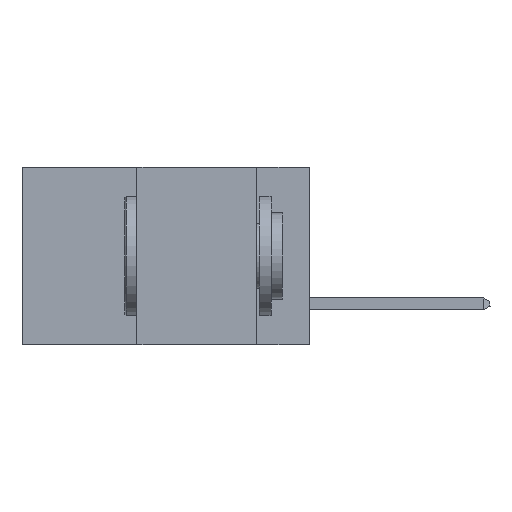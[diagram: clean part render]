
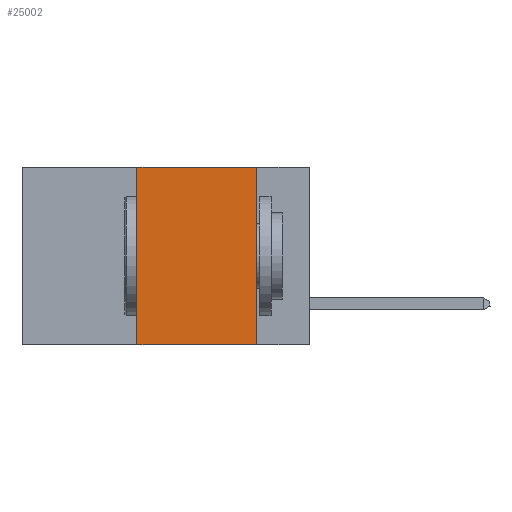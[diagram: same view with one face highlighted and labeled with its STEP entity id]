
A CAD part, left-side view. The second image highlights one B-rep face of the part: STEP entity #25002.
In plain terms, the highlighted planar face has unit normal (-1, 0, 0).
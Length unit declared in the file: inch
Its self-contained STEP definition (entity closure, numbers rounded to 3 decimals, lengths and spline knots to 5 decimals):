
#466 = CARTESIAN_POINT ( 'NONE',  ( 0., 0.6, 0. ) ) ;
#762 = VECTOR ( 'NONE', #21141, 39.37008 ) ;
#1636 = DIRECTION ( 'NONE',  ( 1., 0., 0. ) ) ;
#2012 = VERTEX_POINT ( 'NONE', #11096 ) ;
#3302 = ORIENTED_EDGE ( 'NONE', *, *, #7545, .F. ) ;
#3413 = ORIENTED_EDGE ( 'NONE', *, *, #18417, .F. ) ;
#3528 = VERTEX_POINT ( 'NONE', #21052 ) ;
#3825 = VERTEX_POINT ( 'NONE', #20026 ) ;
#4004 = CARTESIAN_POINT ( 'NONE',  ( 0., 0.6, -0.37 ) ) ;
#4723 = EDGE_LOOP ( 'NONE', ( #3302, #3413, #19471, #14823 ) ) ;
#5394 = LINE ( 'NONE', #10387, #23018 ) ;
#5799 = CARTESIAN_POINT ( 'NONE',  ( 0., 0.6, 0. ) ) ;
#7004 = VECTOR ( 'NONE', #17244, 39.37008 ) ;
#7545 = EDGE_CURVE ( 'NONE', #3528, #3825, #5394, .T. ) ;
#8318 = EDGE_CURVE ( 'NONE', #12825, #2012, #14344, .T. ) ;
#10387 = CARTESIAN_POINT ( 'NONE',  ( 0., 0.11, 0. ) ) ;
#10686 = CARTESIAN_POINT ( 'NONE',  ( 0., 0.36, 0. ) ) ;
#11096 = CARTESIAN_POINT ( 'NONE',  ( 0., 0.36, 0. ) ) ;
#12127 = AXIS2_PLACEMENT_3D ( 'NONE', #5799, #1636, #25105 ) ;
#12825 = VERTEX_POINT ( 'NONE', #22976 ) ;
#13043 = DIRECTION ( 'NONE',  ( 0., 0., -1. ) ) ;
#14344 = LINE ( 'NONE', #10686, #762 ) ;
#14665 = EDGE_CURVE ( 'NONE', #12825, #3825, #14813, .T. ) ;
#14813 = LINE ( 'NONE', #4004, #24074 ) ;
#14823 = ORIENTED_EDGE ( 'NONE', *, *, #14665, .T. ) ;
#17244 = DIRECTION ( 'NONE',  ( 0., -1., 0. ) ) ;
#18417 = EDGE_CURVE ( 'NONE', #2012, #3528, #25944, .T. ) ;
#18541 = PLANE ( 'NONE',  #12127 ) ;
#19419 = FACE_OUTER_BOUND ( 'NONE', #4723, .T. ) ;
#19471 = ORIENTED_EDGE ( 'NONE', *, *, #8318, .F. ) ;
#20026 = CARTESIAN_POINT ( 'NONE',  ( 0., 0.11, -0.37 ) ) ;
#20985 = DIRECTION ( 'NONE',  ( 0., -1., 0. ) ) ;
#21052 = CARTESIAN_POINT ( 'NONE',  ( 0., 0.11, 0. ) ) ;
#21141 = DIRECTION ( 'NONE',  ( 0., 0., 1. ) ) ;
#22976 = CARTESIAN_POINT ( 'NONE',  ( 0., 0.36, -0.37 ) ) ;
#23018 = VECTOR ( 'NONE', #13043, 39.37008 ) ;
#24074 = VECTOR ( 'NONE', #20985, 39.37008 ) ;
#25002 = ADVANCED_FACE ( 'NONE', ( #19419 ), #18541, .F. ) ;
#25105 = DIRECTION ( 'NONE',  ( 0., 0., -1. ) ) ;
#25944 = LINE ( 'NONE', #466, #7004 ) ;
